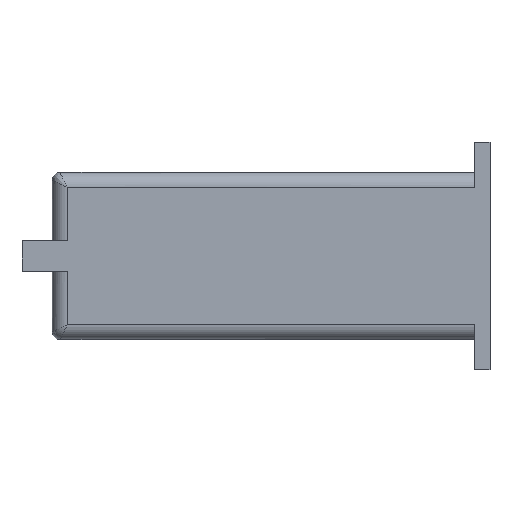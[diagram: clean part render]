
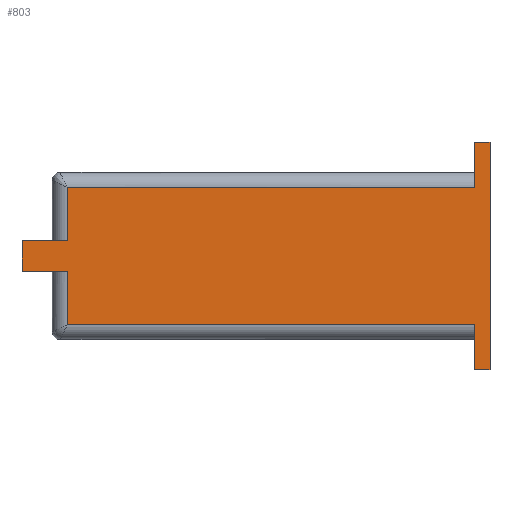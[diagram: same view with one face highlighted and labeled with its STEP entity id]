
A CAD part, top view. The second image highlights one B-rep face of the part: STEP entity #803.
In plain terms, the highlighted planar face has unit normal (0, 0, 1).
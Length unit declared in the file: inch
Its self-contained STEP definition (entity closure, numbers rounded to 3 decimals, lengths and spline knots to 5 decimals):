
#1 = LINE ( 'NONE', #311, #531 ) ;
#5 = CARTESIAN_POINT ( 'NONE',  ( 0., 0., 0.4 ) ) ;
#7 = EDGE_CURVE ( 'NONE', #938, #186, #185, .T. ) ;
#35 = CARTESIAN_POINT ( 'NONE',  ( 5.565, 0., 0.4 ) ) ;
#44 = CARTESIAN_POINT ( 'NONE',  ( 0., -1.3, 0.4 ) ) ;
#46 = DIRECTION ( 'NONE',  ( 0., 1., 0. ) ) ;
#73 = CARTESIAN_POINT ( 'NONE',  ( 0., -2.6, 0.4 ) ) ;
#79 = CARTESIAN_POINT ( 'NONE',  ( -0.4, 0., 0.4 ) ) ;
#82 = CARTESIAN_POINT ( 'NONE',  ( 0., -0.19685, 0.4 ) ) ;
#97 = DIRECTION ( 'NONE',  ( 0., -1., 0. ) ) ;
#98 = VECTOR ( 'NONE', #983, 39.37008 ) ;
#110 = FACE_OUTER_BOUND ( 'NONE', #466, .T. ) ;
#111 = EDGE_CURVE ( 'NONE', #509, #927, #626, .T. ) ;
#148 = ORIENTED_EDGE ( 'NONE', *, *, #563, .T. ) ;
#163 = LINE ( 'NONE', #775, #800 ) ;
#183 = LINE ( 'NONE', #73, #777 ) ;
#185 = LINE ( 'NONE', #44, #912 ) ;
#186 = VERTEX_POINT ( 'NONE', #445 ) ;
#224 = CARTESIAN_POINT ( 'NONE',  ( 0., -0.9, 0.4 ) ) ;
#234 = CARTESIAN_POINT ( 'NONE',  ( -0.4, -0.9, 0.4 ) ) ;
#262 = CARTESIAN_POINT ( 'NONE',  ( 0.19685, -2.00315, 0.4 ) ) ;
#278 = LINE ( 'NONE', #35, #372 ) ;
#282 = ORIENTED_EDGE ( 'NONE', *, *, #353, .T. ) ;
#290 = ORIENTED_EDGE ( 'NONE', *, *, #479, .F. ) ;
#292 = VERTEX_POINT ( 'NONE', #548 ) ;
#295 = ORIENTED_EDGE ( 'NONE', *, *, #631, .F. ) ;
#297 = EDGE_CURVE ( 'NONE', #683, #186, #645, .T. ) ;
#306 = ORIENTED_EDGE ( 'NONE', *, *, #864, .F. ) ;
#311 = CARTESIAN_POINT ( 'NONE',  ( 5.765, 0., 0.4 ) ) ;
#315 = VERTEX_POINT ( 'NONE', #561 ) ;
#344 = LINE ( 'NONE', #485, #757 ) ;
#353 = EDGE_CURVE ( 'NONE', #315, #683, #985, .T. ) ;
#372 = VECTOR ( 'NONE', #46, 39.37008 ) ;
#375 = VERTEX_POINT ( 'NONE', #762 ) ;
#387 = VERTEX_POINT ( 'NONE', #996 ) ;
#388 = DIRECTION ( 'NONE',  ( 1., 0., 0. ) ) ;
#398 = LINE ( 'NONE', #82, #505 ) ;
#416 = CARTESIAN_POINT ( 'NONE',  ( 0.19685, -0.9, 0.4 ) ) ;
#432 = CARTESIAN_POINT ( 'NONE',  ( 5.565, -2.00315, 0.4 ) ) ;
#445 = CARTESIAN_POINT ( 'NONE',  ( -0.4, -1.3, 0.4 ) ) ;
#466 = EDGE_LOOP ( 'NONE', ( #306, #295, #290, #988, #569, #282, #665, #545, #148, #547, #636, #1001 ) ) ;
#479 = EDGE_CURVE ( 'NONE', #375, #831, #278, .T. ) ;
#485 = CARTESIAN_POINT ( 'NONE',  ( 5.565, 0., 0.4 ) ) ;
#505 = VECTOR ( 'NONE', #633, 39.37008 ) ;
#509 = VERTEX_POINT ( 'NONE', #262 ) ;
#531 = VECTOR ( 'NONE', #559, 39.37008 ) ;
#541 = DIRECTION ( 'NONE',  ( 1., 0., 0. ) ) ;
#545 = ORIENTED_EDGE ( 'NONE', *, *, #7, .F. ) ;
#547 = ORIENTED_EDGE ( 'NONE', *, *, #111, .T. ) ;
#548 = CARTESIAN_POINT ( 'NONE',  ( 5.765, 0.4, 0.4 ) ) ;
#559 = DIRECTION ( 'NONE',  ( 0., -1., 0. ) ) ;
#561 = CARTESIAN_POINT ( 'NONE',  ( 0.19685, -0.9, 0.4 ) ) ;
#562 = CARTESIAN_POINT ( 'NONE',  ( 5.565, -2.00315, 0.4 ) ) ;
#563 = EDGE_CURVE ( 'NONE', #938, #509, #625, .T. ) ;
#569 = ORIENTED_EDGE ( 'NONE', *, *, #978, .T. ) ;
#590 = EDGE_CURVE ( 'NONE', #387, #772, #183, .T. ) ;
#595 = DIRECTION ( 'NONE',  ( -1., 0., 0. ) ) ;
#625 = LINE ( 'NONE', #664, #98 ) ;
#626 = LINE ( 'NONE', #432, #884 ) ;
#631 = EDGE_CURVE ( 'NONE', #831, #292, #163, .T. ) ;
#633 = DIRECTION ( 'NONE',  ( -1., 0., 0. ) ) ;
#636 = ORIENTED_EDGE ( 'NONE', *, *, #939, .T. ) ;
#637 = DIRECTION ( 'NONE',  ( 0., -1., 0. ) ) ;
#645 = LINE ( 'NONE', #79, #662 ) ;
#662 = VECTOR ( 'NONE', #97, 39.37008 ) ;
#664 = CARTESIAN_POINT ( 'NONE',  ( 0.19685, -2.2, 0.4 ) ) ;
#665 = ORIENTED_EDGE ( 'NONE', *, *, #297, .T. ) ;
#682 = PLANE ( 'NONE',  #847 ) ;
#683 = VERTEX_POINT ( 'NONE', #234 ) ;
#693 = DIRECTION ( 'NONE',  ( 0., 0., 1. ) ) ;
#757 = VECTOR ( 'NONE', #637, 39.37008 ) ;
#762 = CARTESIAN_POINT ( 'NONE',  ( 5.565, -0.19685, 0.4 ) ) ;
#768 = VECTOR ( 'NONE', #769, 39.37008 ) ;
#769 = DIRECTION ( 'NONE',  ( -1., 0., 0. ) ) ;
#772 = VERTEX_POINT ( 'NONE', #968 ) ;
#775 = CARTESIAN_POINT ( 'NONE',  ( 0., 0.4, 0.4 ) ) ;
#777 = VECTOR ( 'NONE', #541, 39.37008 ) ;
#780 = VECTOR ( 'NONE', #953, 39.37008 ) ;
#800 = VECTOR ( 'NONE', #388, 39.37008 ) ;
#803 = ADVANCED_FACE ( 'NONE', ( #110 ), #682, .T. ) ;
#831 = VERTEX_POINT ( 'NONE', #839 ) ;
#832 = LINE ( 'NONE', #416, #780 ) ;
#839 = CARTESIAN_POINT ( 'NONE',  ( 5.565, 0.4, 0.4 ) ) ;
#845 = VERTEX_POINT ( 'NONE', #854 ) ;
#847 = AXIS2_PLACEMENT_3D ( 'NONE', #5, #693, #995 ) ;
#854 = CARTESIAN_POINT ( 'NONE',  ( 0.19685, -0.19685, 0.4 ) ) ;
#856 = CARTESIAN_POINT ( 'NONE',  ( 0.19685, -1.3, 0.4 ) ) ;
#864 = EDGE_CURVE ( 'NONE', #292, #772, #1, .T. ) ;
#884 = VECTOR ( 'NONE', #969, 39.37008 ) ;
#906 = EDGE_CURVE ( 'NONE', #375, #845, #398, .T. ) ;
#912 = VECTOR ( 'NONE', #595, 39.37008 ) ;
#927 = VERTEX_POINT ( 'NONE', #562 ) ;
#938 = VERTEX_POINT ( 'NONE', #856 ) ;
#939 = EDGE_CURVE ( 'NONE', #927, #387, #344, .T. ) ;
#953 = DIRECTION ( 'NONE',  ( 0., -1., 0. ) ) ;
#968 = CARTESIAN_POINT ( 'NONE',  ( 5.765, -2.6, 0.4 ) ) ;
#969 = DIRECTION ( 'NONE',  ( 1., 0., 0. ) ) ;
#978 = EDGE_CURVE ( 'NONE', #845, #315, #832, .T. ) ;
#983 = DIRECTION ( 'NONE',  ( 0., -1., 0. ) ) ;
#985 = LINE ( 'NONE', #224, #768 ) ;
#988 = ORIENTED_EDGE ( 'NONE', *, *, #906, .T. ) ;
#995 = DIRECTION ( 'NONE',  ( 1., 0., 0. ) ) ;
#996 = CARTESIAN_POINT ( 'NONE',  ( 5.565, -2.6, 0.4 ) ) ;
#1001 = ORIENTED_EDGE ( 'NONE', *, *, #590, .T. ) ;
